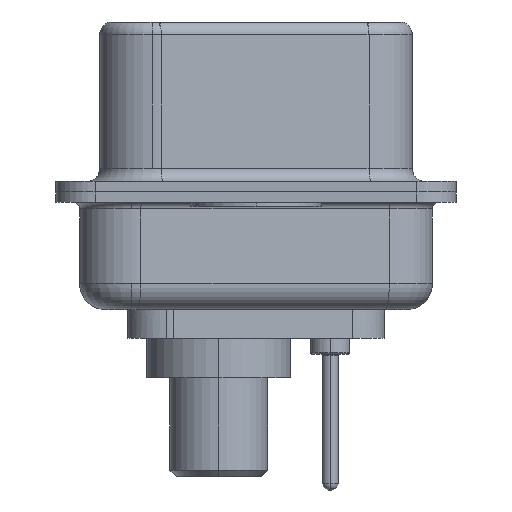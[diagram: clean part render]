
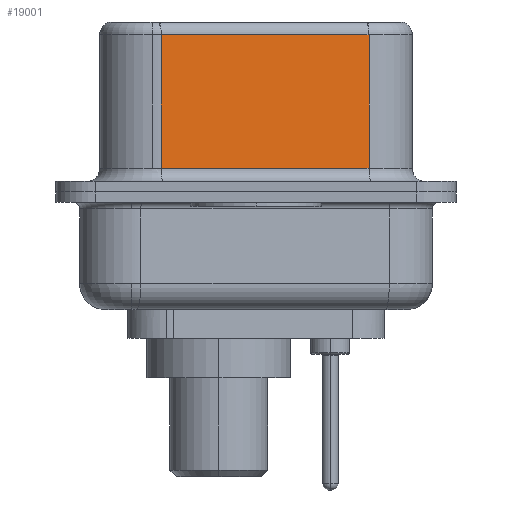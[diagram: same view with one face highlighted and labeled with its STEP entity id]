
A CAD part, left-side view. The second image highlights one B-rep face of the part: STEP entity #19001.
In plain terms, the highlighted planar face has unit normal (-0.985, -0.174, 0).
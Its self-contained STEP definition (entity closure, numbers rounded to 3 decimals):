
#82 = VECTOR ( 'NONE', #6621, 1000. ) ;
#462 = VERTEX_POINT ( 'NONE', #8257 ) ;
#601 = LINE ( 'NONE', #9552, #82 ) ;
#2763 = PLANE ( 'NONE',  #17896 ) ;
#2812 = EDGE_CURVE ( 'NONE', #462, #16514, #16730, .T. ) ;
#2881 = ORIENTED_EDGE ( 'NONE', *, *, #13499, .F. ) ;
#3027 = DIRECTION ( 'NONE',  ( -0.174, 0.985, 0. ) ) ;
#3879 = VECTOR ( 'NONE', #3027, 1000. ) ;
#4420 = CARTESIAN_POINT ( 'NONE',  ( 5.132, -4.322, 0.9 ) ) ;
#4809 = VECTOR ( 'NONE', #12185, 1000. ) ;
#5628 = ORIENTED_EDGE ( 'NONE', *, *, #2812, .T. ) ;
#6171 = EDGE_LOOP ( 'NONE', ( #2881, #13101, #5628, #8513 ) ) ;
#6621 = DIRECTION ( 'NONE',  ( 0., 0., -1. ) ) ;
#7206 = CARTESIAN_POINT ( 'NONE',  ( 5.132, -4.322, 6.02 ) ) ;
#7742 = CARTESIAN_POINT ( 'NONE',  ( 5.132, -4.322, 0.9 ) ) ;
#7832 = CARTESIAN_POINT ( 'NONE',  ( 3.73, 3.628, 0.9 ) ) ;
#8257 = CARTESIAN_POINT ( 'NONE',  ( 3.73, 3.628, 6.02 ) ) ;
#8513 = ORIENTED_EDGE ( 'NONE', *, *, #11510, .T. ) ;
#8778 = CARTESIAN_POINT ( 'NONE',  ( 5.132, -4.322, 6.52 ) ) ;
#8798 = VERTEX_POINT ( 'NONE', #7206 ) ;
#8815 = FACE_OUTER_BOUND ( 'NONE', #6171, .T. ) ;
#9247 = DIRECTION ( 'NONE',  ( 0.174, -0.985, 0. ) ) ;
#9552 = CARTESIAN_POINT ( 'NONE',  ( 5.132, -4.322, 6.52 ) ) ;
#9573 = VECTOR ( 'NONE', #9247, 1000. ) ;
#9803 = CARTESIAN_POINT ( 'NONE',  ( 3.73, 3.628, 6.52 ) ) ;
#10272 = DIRECTION ( 'NONE',  ( -0.174, 0.985, 0. ) ) ;
#11372 = LINE ( 'NONE', #11969, #3879 ) ;
#11510 = EDGE_CURVE ( 'NONE', #16514, #14306, #17526, .T. ) ;
#11969 = CARTESIAN_POINT ( 'NONE',  ( 5.132, -4.322, 6.02 ) ) ;
#12185 = DIRECTION ( 'NONE',  ( 0., 0., -1. ) ) ;
#13101 = ORIENTED_EDGE ( 'NONE', *, *, #13751, .T. ) ;
#13499 = EDGE_CURVE ( 'NONE', #8798, #14306, #601, .T. ) ;
#13751 = EDGE_CURVE ( 'NONE', #8798, #462, #11372, .T. ) ;
#14306 = VERTEX_POINT ( 'NONE', #4420 ) ;
#16514 = VERTEX_POINT ( 'NONE', #7832 ) ;
#16730 = LINE ( 'NONE', #9803, #4809 ) ;
#17526 = LINE ( 'NONE', #7742, #9573 ) ;
#17896 = AXIS2_PLACEMENT_3D ( 'NONE', #8778, #19153, #10272 ) ;
#19001 = ADVANCED_FACE ( 'NONE', ( #8815 ), #2763, .F. ) ;
#19153 = DIRECTION ( 'NONE',  ( 0.985, 0.174, 0. ) ) ;
